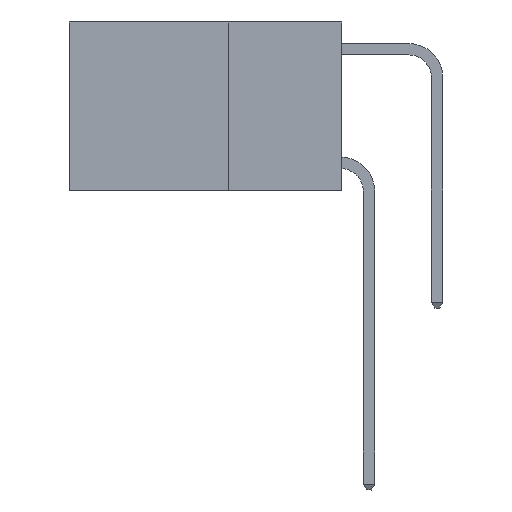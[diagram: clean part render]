
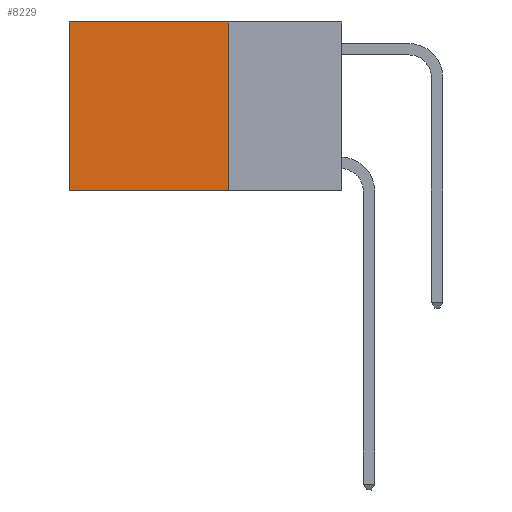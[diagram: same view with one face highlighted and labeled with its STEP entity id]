
A CAD part, left-side view. The second image highlights one B-rep face of the part: STEP entity #8229.
In plain terms, the highlighted planar face has unit normal (-1, 0, 0).
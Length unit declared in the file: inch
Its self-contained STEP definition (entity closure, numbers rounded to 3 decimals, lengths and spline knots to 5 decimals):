
#720 = VECTOR ( 'NONE', #3003, 39.37008 ) ;
#786 = LINE ( 'NONE', #5539, #11159 ) ;
#1033 = EDGE_CURVE ( 'NONE', #5585, #5568, #786, .T. ) ;
#1151 = PLANE ( 'NONE',  #9772 ) ;
#1198 = CARTESIAN_POINT ( 'NONE',  ( 0.2625, 0.6, 0. ) ) ;
#2158 = DIRECTION ( 'NONE',  ( 0., 0., -1. ) ) ;
#2400 = CARTESIAN_POINT ( 'NONE',  ( 0.2625, 0.25, 0. ) ) ;
#2414 = ORIENTED_EDGE ( 'NONE', *, *, #7806, .T. ) ;
#2438 = VERTEX_POINT ( 'NONE', #8754 ) ;
#3003 = DIRECTION ( 'NONE',  ( 0., 0., -1. ) ) ;
#3384 = ORIENTED_EDGE ( 'NONE', *, *, #1033, .F. ) ;
#3541 = CARTESIAN_POINT ( 'NONE',  ( 0.2625, 0.25, -0.37 ) ) ;
#3882 = DIRECTION ( 'NONE',  ( 0., 0., -1. ) ) ;
#4372 = CARTESIAN_POINT ( 'NONE',  ( 0.2625, 0.6, -0.37 ) ) ;
#4962 = VECTOR ( 'NONE', #3882, 39.37008 ) ;
#5082 = EDGE_LOOP ( 'NONE', ( #2414, #3384, #9363, #6862 ) ) ;
#5367 = VECTOR ( 'NONE', #11309, 39.37008 ) ;
#5419 = EDGE_CURVE ( 'NONE', #2438, #5585, #9130, .T. ) ;
#5539 = CARTESIAN_POINT ( 'NONE',  ( 0.2625, 0.25, -0.37 ) ) ;
#5568 = VERTEX_POINT ( 'NONE', #4372 ) ;
#5585 = VERTEX_POINT ( 'NONE', #3541 ) ;
#6031 = EDGE_CURVE ( 'NONE', #2438, #9987, #9938, .T. ) ;
#6862 = ORIENTED_EDGE ( 'NONE', *, *, #6031, .T. ) ;
#7526 = DIRECTION ( 'NONE',  ( 0., 1., 0. ) ) ;
#7806 = EDGE_CURVE ( 'NONE', #9987, #5568, #10972, .T. ) ;
#8079 = FACE_OUTER_BOUND ( 'NONE', #5082, .T. ) ;
#8229 = ADVANCED_FACE ( 'NONE', ( #8079 ), #1151, .F. ) ;
#8754 = CARTESIAN_POINT ( 'NONE',  ( 0.2625, 0.25, 0. ) ) ;
#9019 = CARTESIAN_POINT ( 'NONE',  ( 0.2625, 0.25, 0. ) ) ;
#9055 = CARTESIAN_POINT ( 'NONE',  ( 0.2625, 0.25, 0. ) ) ;
#9130 = LINE ( 'NONE', #2400, #4962 ) ;
#9363 = ORIENTED_EDGE ( 'NONE', *, *, #5419, .F. ) ;
#9772 = AXIS2_PLACEMENT_3D ( 'NONE', #9019, #9952, #2158 ) ;
#9918 = CARTESIAN_POINT ( 'NONE',  ( 0.2625, 0.6, 0. ) ) ;
#9938 = LINE ( 'NONE', #9055, #5367 ) ;
#9952 = DIRECTION ( 'NONE',  ( 1., 0., 0. ) ) ;
#9987 = VERTEX_POINT ( 'NONE', #1198 ) ;
#10972 = LINE ( 'NONE', #9918, #720 ) ;
#11159 = VECTOR ( 'NONE', #7526, 39.37008 ) ;
#11309 = DIRECTION ( 'NONE',  ( 0., 1., 0. ) ) ;
